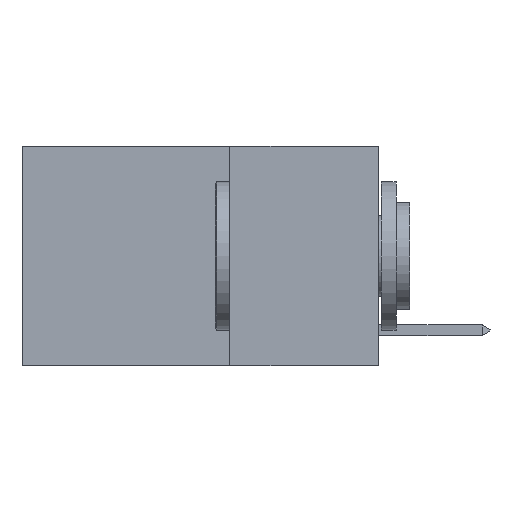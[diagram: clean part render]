
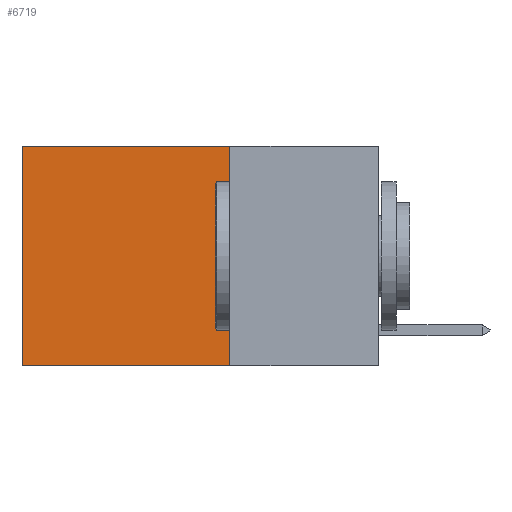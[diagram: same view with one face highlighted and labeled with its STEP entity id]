
A CAD part, left-side view. The second image highlights one B-rep face of the part: STEP entity #6719.
In plain terms, the highlighted planar face has unit normal (-1, 0, 0).
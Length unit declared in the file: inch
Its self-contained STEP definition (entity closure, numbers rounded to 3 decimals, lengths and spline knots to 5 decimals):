
#1098 = CARTESIAN_POINT ( 'NONE',  ( 0.2625, 0.25, 0. ) ) ;
#1247 = ORIENTED_EDGE ( 'NONE', *, *, #30115, .T. ) ;
#2050 = EDGE_CURVE ( 'NONE', #11144, #23155, #25588, .T. ) ;
#2347 = DIRECTION ( 'NONE',  ( 0., 0., -1. ) ) ;
#5677 = AXIS2_PLACEMENT_3D ( 'NONE', #1098, #24155, #21729 ) ;
#5895 = ORIENTED_EDGE ( 'NONE', *, *, #24055, .F. ) ;
#5975 = LINE ( 'NONE', #12988, #18383 ) ;
#5985 = VERTEX_POINT ( 'NONE', #30033 ) ;
#6719 = ADVANCED_FACE ( 'NONE', ( #20487 ), #7983, .F. ) ;
#7090 = CARTESIAN_POINT ( 'NONE',  ( 0.2625, 0.25, 0. ) ) ;
#7983 = PLANE ( 'NONE',  #5677 ) ;
#8229 = DIRECTION ( 'NONE',  ( 0., 1., 0. ) ) ;
#8805 = CARTESIAN_POINT ( 'NONE',  ( 0.2625, 0.25, -0.37 ) ) ;
#9068 = VECTOR ( 'NONE', #8229, 39.37008 ) ;
#10554 = DIRECTION ( 'NONE',  ( 0., 1., 0. ) ) ;
#11144 = VERTEX_POINT ( 'NONE', #30176 ) ;
#11409 = EDGE_LOOP ( 'NONE', ( #16559, #5895, #14168, #1247 ) ) ;
#12129 = VECTOR ( 'NONE', #16305, 39.37008 ) ;
#12988 = CARTESIAN_POINT ( 'NONE',  ( 0.2625, 0.25, -0.37 ) ) ;
#13141 = VERTEX_POINT ( 'NONE', #8805 ) ;
#14168 = ORIENTED_EDGE ( 'NONE', *, *, #20785, .F. ) ;
#15266 = CARTESIAN_POINT ( 'NONE',  ( 0.2625, 0.25, 0. ) ) ;
#15311 = VECTOR ( 'NONE', #2347, 39.37008 ) ;
#16305 = DIRECTION ( 'NONE',  ( 0., 0., -1. ) ) ;
#16559 = ORIENTED_EDGE ( 'NONE', *, *, #2050, .T. ) ;
#18383 = VECTOR ( 'NONE', #10554, 39.37008 ) ;
#20487 = FACE_OUTER_BOUND ( 'NONE', #11409, .T. ) ;
#20785 = EDGE_CURVE ( 'NONE', #5985, #13141, #23273, .T. ) ;
#21729 = DIRECTION ( 'NONE',  ( 0., 0., -1. ) ) ;
#23155 = VERTEX_POINT ( 'NONE', #23795 ) ;
#23273 = LINE ( 'NONE', #7090, #15311 ) ;
#23795 = CARTESIAN_POINT ( 'NONE',  ( 0.2625, 0.6, -0.37 ) ) ;
#24055 = EDGE_CURVE ( 'NONE', #13141, #23155, #5975, .T. ) ;
#24094 = LINE ( 'NONE', #15266, #9068 ) ;
#24155 = DIRECTION ( 'NONE',  ( 1., 0., 0. ) ) ;
#25588 = LINE ( 'NONE', #29882, #12129 ) ;
#29882 = CARTESIAN_POINT ( 'NONE',  ( 0.2625, 0.6, 0. ) ) ;
#30033 = CARTESIAN_POINT ( 'NONE',  ( 0.2625, 0.25, 0. ) ) ;
#30115 = EDGE_CURVE ( 'NONE', #5985, #11144, #24094, .T. ) ;
#30176 = CARTESIAN_POINT ( 'NONE',  ( 0.2625, 0.6, 0. ) ) ;
